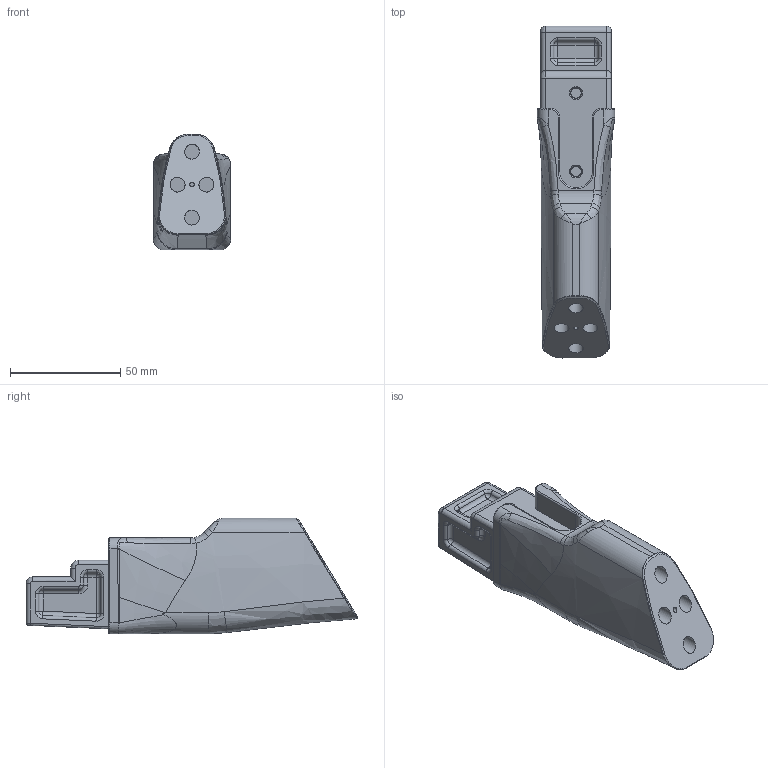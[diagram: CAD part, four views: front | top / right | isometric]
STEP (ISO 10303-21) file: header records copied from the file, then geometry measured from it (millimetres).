
FILE_DESCRIPTION(/* description */ (''),/* implementation_level */ '2;1');
FILE_NAME(/* name */ 'Stock Half 2.step',/* time_stamp */ '2021-10-03T07:00:28-04:00',/* author */ (''),/* organization */ (''),/* preprocessor_version */ 'ST-DEVELOPER v18.1',/* originating_system */ 'Autodesk Translation Framework v10.10.0.1391',/* authorisation */ '');
FILE_SCHEMA (('AUTOMOTIVE_DESIGN { 1 0 10303 214 3 1 1 }'));
Length unit declared in the file: millimetre
Products named in the file (1): Stock Half 2
Bounding box: 35 x 150.22 x 52.44 mm (x, y, z)
Volume: 122520.6 mm3; surface area: 28615.3 mm2
Topology: 1 solids, 1 shells, 286 faces, 656 edges, 379 vertices
Faces by surface type: cylinder 101, bspline 92, plane 34, torus 33, sphere 24, cone 2
Full cylindrical faces by diameter (mm): 2 x1, 4.6 x2, 6.7 x4
Entity records: 10187 total; most frequent: CARTESIAN_POINT 4111, ORIENTED_EDGE 1300, DIRECTION 1197, EDGE_CURVE 650, AXIS2_PLACEMENT_3D 503, VERTEX_POINT 379, EDGE_LOOP 299, FACE_OUTER_BOUND 286
